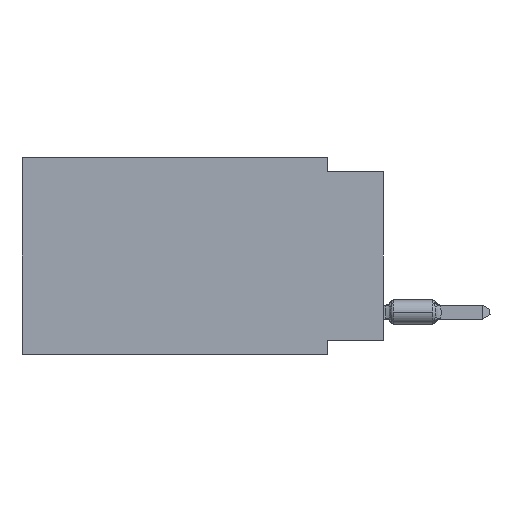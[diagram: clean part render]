
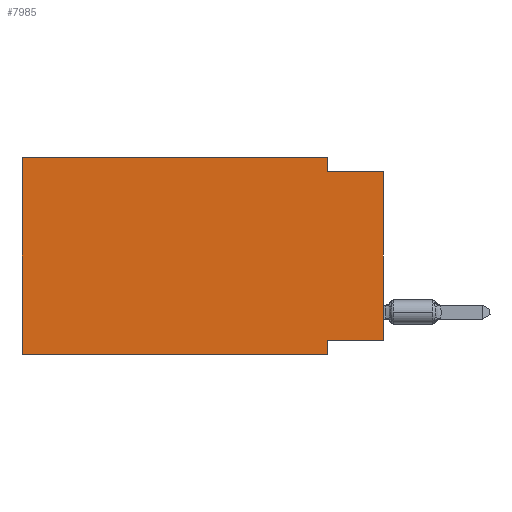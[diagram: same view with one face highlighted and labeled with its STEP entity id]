
A CAD part, left-side view. The second image highlights one B-rep face of the part: STEP entity #7985.
In plain terms, the highlighted planar face has unit normal (-1, 0, 0).
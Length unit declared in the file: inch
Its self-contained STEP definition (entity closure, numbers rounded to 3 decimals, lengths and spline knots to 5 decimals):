
#939 = ORIENTED_EDGE ( 'NONE', *, *, #9820, .F. ) ;
#1338 = EDGE_CURVE ( 'NONE', #36049, #33040, #20687, .T. ) ;
#1339 = VERTEX_POINT ( 'NONE', #29720 ) ;
#3316 = DIRECTION ( 'NONE',  ( 0., 0., -1. ) ) ;
#3968 = EDGE_LOOP ( 'NONE', ( #4901, #30869, #16543, #20965, #17795, #11887, #20319, #939 ) ) ;
#4780 = CARTESIAN_POINT ( 'NONE',  ( 0., 0., -0.325 ) ) ;
#4901 = ORIENTED_EDGE ( 'NONE', *, *, #5038, .T. ) ;
#5038 = EDGE_CURVE ( 'NONE', #1339, #12887, #9883, .T. ) ;
#6191 = DIRECTION ( 'NONE',  ( 0., -1., 0. ) ) ;
#6705 = VECTOR ( 'NONE', #29102, 39.37008 ) ;
#7633 = VECTOR ( 'NONE', #31010, 39.37008 ) ;
#7696 = VECTOR ( 'NONE', #18613, 39.37008 ) ;
#7985 = ADVANCED_FACE ( 'NONE', ( #29407 ), #31844, .F. ) ;
#8087 = DIRECTION ( 'NONE',  ( 0., 0., -1. ) ) ;
#8219 = DIRECTION ( 'NONE',  ( 0., 0., 1. ) ) ;
#9210 = CARTESIAN_POINT ( 'NONE',  ( 0., 0.645, 0. ) ) ;
#9364 = LINE ( 'NONE', #25223, #7696 ) ;
#9820 = EDGE_CURVE ( 'NONE', #1339, #15175, #16850, .T. ) ;
#9883 = LINE ( 'NONE', #22160, #26596 ) ;
#10783 = CARTESIAN_POINT ( 'NONE',  ( 0., 0.1, 0. ) ) ;
#10932 = VECTOR ( 'NONE', #3316, 39.37008 ) ;
#11887 = ORIENTED_EDGE ( 'NONE', *, *, #28118, .T. ) ;
#12887 = VERTEX_POINT ( 'NONE', #25348 ) ;
#13672 = VERTEX_POINT ( 'NONE', #39551 ) ;
#13749 = DIRECTION ( 'NONE',  ( 1., 0., 0. ) ) ;
#15175 = VERTEX_POINT ( 'NONE', #35628 ) ;
#15768 = EDGE_CURVE ( 'NONE', #25205, #36049, #35772, .T. ) ;
#16349 = CARTESIAN_POINT ( 'NONE',  ( 0., 0.645, 0. ) ) ;
#16543 = ORIENTED_EDGE ( 'NONE', *, *, #21886, .F. ) ;
#16850 = LINE ( 'NONE', #4780, #6705 ) ;
#17795 = ORIENTED_EDGE ( 'NONE', *, *, #15768, .F. ) ;
#18613 = DIRECTION ( 'NONE',  ( 0., -1., 0. ) ) ;
#19146 = DIRECTION ( 'NONE',  ( 0., 0., 1. ) ) ;
#19524 = VERTEX_POINT ( 'NONE', #30203 ) ;
#20319 = ORIENTED_EDGE ( 'NONE', *, *, #29243, .F. ) ;
#20687 = LINE ( 'NONE', #9210, #35038 ) ;
#20965 = ORIENTED_EDGE ( 'NONE', *, *, #1338, .F. ) ;
#21886 = EDGE_CURVE ( 'NONE', #33040, #13672, #26392, .T. ) ;
#22160 = CARTESIAN_POINT ( 'NONE',  ( 0., 0., 0. ) ) ;
#23918 = CARTESIAN_POINT ( 'NONE',  ( 0., 0.645, 0. ) ) ;
#25205 = VERTEX_POINT ( 'NONE', #28399 ) ;
#25223 = CARTESIAN_POINT ( 'NONE',  ( 0., 0., -0.025 ) ) ;
#25348 = CARTESIAN_POINT ( 'NONE',  ( 0., 0., -0.025 ) ) ;
#26392 = LINE ( 'NONE', #35642, #35036 ) ;
#26596 = VECTOR ( 'NONE', #19146, 39.37008 ) ;
#27196 = LINE ( 'NONE', #39469, #7633 ) ;
#28118 = EDGE_CURVE ( 'NONE', #25205, #19524, #27196, .T. ) ;
#28399 = CARTESIAN_POINT ( 'NONE',  ( 0., 0.645, -0.35 ) ) ;
#29102 = DIRECTION ( 'NONE',  ( 0., 1., 0. ) ) ;
#29243 = EDGE_CURVE ( 'NONE', #15175, #19524, #30469, .T. ) ;
#29407 = FACE_OUTER_BOUND ( 'NONE', #3968, .T. ) ;
#29720 = CARTESIAN_POINT ( 'NONE',  ( 0., 0., -0.325 ) ) ;
#30203 = CARTESIAN_POINT ( 'NONE',  ( 0., 0.1, -0.35 ) ) ;
#30469 = LINE ( 'NONE', #30858, #10932 ) ;
#30858 = CARTESIAN_POINT ( 'NONE',  ( 0., 0.1, -0.35 ) ) ;
#30869 = ORIENTED_EDGE ( 'NONE', *, *, #39468, .F. ) ;
#31010 = DIRECTION ( 'NONE',  ( 0., -1., 0. ) ) ;
#31844 = PLANE ( 'NONE',  #36107 ) ;
#32604 = VECTOR ( 'NONE', #8219, 39.37008 ) ;
#33040 = VERTEX_POINT ( 'NONE', #10783 ) ;
#35036 = VECTOR ( 'NONE', #8087, 39.37008 ) ;
#35038 = VECTOR ( 'NONE', #6191, 39.37008 ) ;
#35237 = CARTESIAN_POINT ( 'NONE',  ( 0., 0.645, 0. ) ) ;
#35628 = CARTESIAN_POINT ( 'NONE',  ( 0., 0.1, -0.325 ) ) ;
#35642 = CARTESIAN_POINT ( 'NONE',  ( 0., 0.1, 0. ) ) ;
#35772 = LINE ( 'NONE', #23918, #32604 ) ;
#36049 = VERTEX_POINT ( 'NONE', #16349 ) ;
#36107 = AXIS2_PLACEMENT_3D ( 'NONE', #35237, #13749, #38463 ) ;
#38463 = DIRECTION ( 'NONE',  ( 0., 0., -1. ) ) ;
#39468 = EDGE_CURVE ( 'NONE', #13672, #12887, #9364, .T. ) ;
#39469 = CARTESIAN_POINT ( 'NONE',  ( 0., 0.645, -0.35 ) ) ;
#39551 = CARTESIAN_POINT ( 'NONE',  ( 0., 0.1, -0.025 ) ) ;
